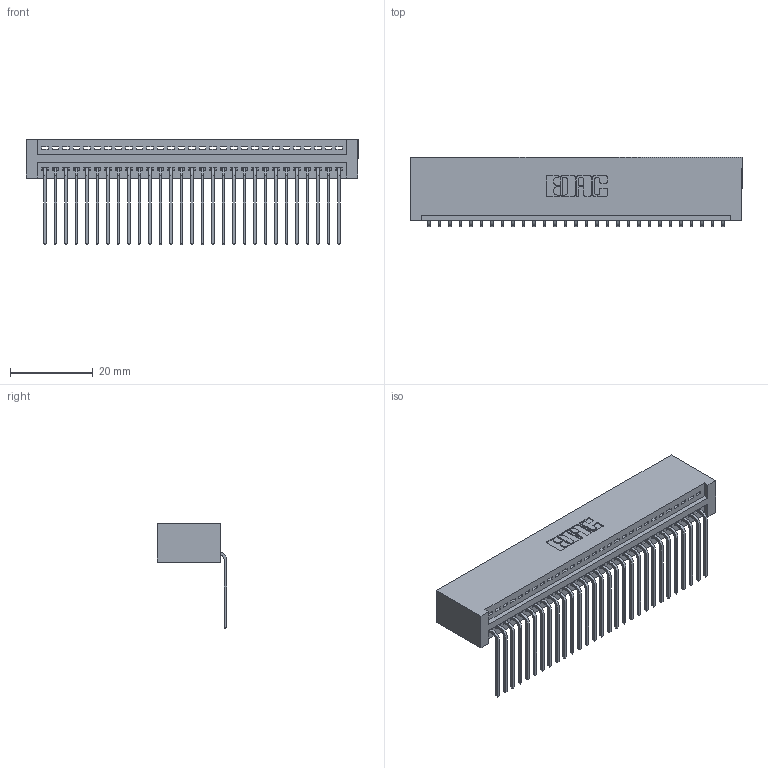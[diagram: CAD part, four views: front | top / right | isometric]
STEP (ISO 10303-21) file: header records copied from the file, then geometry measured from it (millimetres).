
FILE_DESCRIPTION (( 'STEP AP203' ), '1' );
FILE_NAME ('395-029-559-101.STEP', '2018-11-10T21:47:23', ( '' ), ( '' ), 'SwSTEP 2.0', 'SolidWorks 2016', '' );
FILE_SCHEMA (( 'CONFIG_CONTROL_DESIGN' ));
Length unit declared in the file: inch
Products named in the file (3): 395-029-559-101; 345 Part_No Mounting Lugs; 345-292-001_558 559 Tail - 1
Assembly tree (30 placements, depth 2):
  395-029-559-101
    345 Part_No Mounting Lugs
    345-292-001_558 559 Tail - 1  x29
Bounding box: 80.26 x 16.75 x 25.53 mm (x, y, z)
Volume: 8198 mm3; surface area: 11475.7 mm2
Topology: 30 solids, 30 shells, 1858 faces, 5595 edges, 3690 vertices
Faces by surface type: plane 1294, cylinder 564
Entity records: 23383 total; most frequent: CARTESIAN_POINT 4059, ORIENTED_EDGE 4022, DIRECTION 3557, EDGE_CURVE 2011, VECTOR 1771, LINE 1771, VERTEX_POINT 1338, AXIS2_PLACEMENT_3D 893
